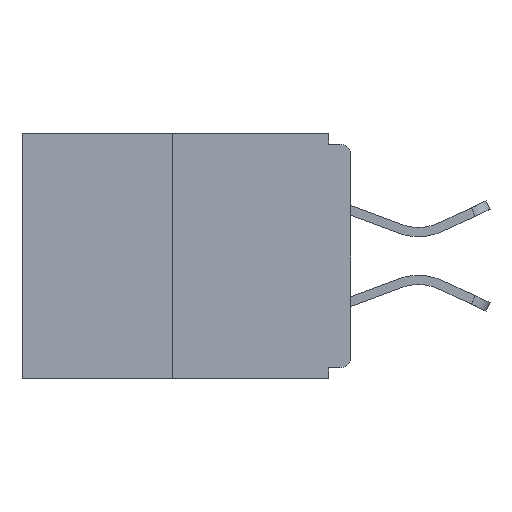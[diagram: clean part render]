
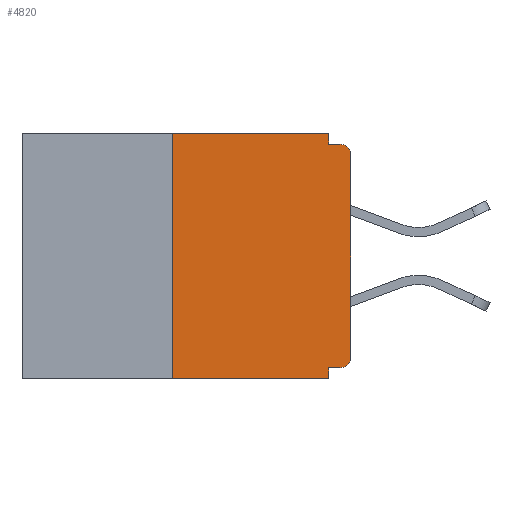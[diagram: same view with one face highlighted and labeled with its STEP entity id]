
A CAD part, left-side view. The second image highlights one B-rep face of the part: STEP entity #4820.
In plain terms, the highlighted planar face has unit normal (-1, 0, 0).
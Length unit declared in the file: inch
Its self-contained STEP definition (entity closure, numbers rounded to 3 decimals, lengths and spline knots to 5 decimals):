
#71 = LINE ( 'NONE', #4226, #3822 ) ;
#185 = VECTOR ( 'NONE', #7769, 39.37008 ) ;
#435 = EDGE_CURVE ( 'NONE', #2925, #9922, #7428, .T. ) ;
#478 = ORIENTED_EDGE ( 'NONE', *, *, #12668, .T. ) ;
#519 = VERTEX_POINT ( 'NONE', #4564 ) ;
#611 = ORIENTED_EDGE ( 'NONE', *, *, #435, .T. ) ;
#626 = CARTESIAN_POINT ( 'NONE',  ( 0., 0.46, -0.343 ) ) ;
#725 = ORIENTED_EDGE ( 'NONE', *, *, #7886, .F. ) ;
#737 = VECTOR ( 'NONE', #5332, 39.37008 ) ;
#765 = DIRECTION ( 'NONE',  ( 0., 0., -1. ) ) ;
#860 = DIRECTION ( 'NONE',  ( 1., 0., 0. ) ) ;
#923 = ORIENTED_EDGE ( 'NONE', *, *, #10808, .F. ) ;
#1026 = CARTESIAN_POINT ( 'NONE',  ( 0., 0., -0.03 ) ) ;
#1779 = EDGE_CURVE ( 'NONE', #11652, #10095, #10663, .T. ) ;
#2315 = DIRECTION ( 'NONE',  ( 0., -1., 0. ) ) ;
#2351 = EDGE_CURVE ( 'NONE', #9922, #11652, #6791, .T. ) ;
#2826 = EDGE_LOOP ( 'NONE', ( #10183, #725, #478, #5911, #923, #611, #11183, #9332, #3282, #5860 ) ) ;
#2859 = CARTESIAN_POINT ( 'NONE',  ( 0., 0.031, 0. ) ) ;
#2925 = VERTEX_POINT ( 'NONE', #9505 ) ;
#2957 = FACE_OUTER_BOUND ( 'NONE', #2826, .T. ) ;
#3062 = AXIS2_PLACEMENT_3D ( 'NONE', #10218, #860, #7151 ) ;
#3282 = ORIENTED_EDGE ( 'NONE', *, *, #10199, .F. ) ;
#3587 = CARTESIAN_POINT ( 'NONE',  ( 0., 0., -0.313 ) ) ;
#3663 = DIRECTION ( 'NONE',  ( 0., -1., 0. ) ) ;
#3822 = VECTOR ( 'NONE', #7380, 39.37008 ) ;
#3829 = CARTESIAN_POINT ( 'NONE',  ( 0., 0.031, -0.343 ) ) ;
#3863 = VERTEX_POINT ( 'NONE', #10115 ) ;
#3864 = EDGE_CURVE ( 'NONE', #519, #10175, #6966, .T. ) ;
#4024 = DIRECTION ( 'NONE',  ( 0., 0., -1. ) ) ;
#4149 = CARTESIAN_POINT ( 'NONE',  ( 0., 0.031, -0.328 ) ) ;
#4226 = CARTESIAN_POINT ( 'NONE',  ( 0., 0., -0.015 ) ) ;
#4564 = CARTESIAN_POINT ( 'NONE',  ( 0., 0.031, 0. ) ) ;
#4583 = CARTESIAN_POINT ( 'NONE',  ( 0., 0.46, 0. ) ) ;
#4603 = CARTESIAN_POINT ( 'NONE',  ( 0., 0., -0.328 ) ) ;
#4730 = VECTOR ( 'NONE', #3663, 39.37008 ) ;
#4741 = LINE ( 'NONE', #4603, #7760 ) ;
#4764 = AXIS2_PLACEMENT_3D ( 'NONE', #7542, #11689, #12145 ) ;
#4820 = ADVANCED_FACE ( 'NONE', ( #2957 ), #12244, .F. ) ;
#5332 = DIRECTION ( 'NONE',  ( 0., 0., 1. ) ) ;
#5860 = ORIENTED_EDGE ( 'NONE', *, *, #3864, .F. ) ;
#5911 = ORIENTED_EDGE ( 'NONE', *, *, #7331, .F. ) ;
#6486 = VERTEX_POINT ( 'NONE', #4149 ) ;
#6642 = CARTESIAN_POINT ( 'NONE',  ( 0., 0.25, 0. ) ) ;
#6791 = LINE ( 'NONE', #9806, #185 ) ;
#6966 = LINE ( 'NONE', #2859, #11855 ) ;
#6979 = DIRECTION ( 'NONE',  ( 0., 0., -1. ) ) ;
#7151 = DIRECTION ( 'NONE',  ( 0., 0., -1. ) ) ;
#7331 = EDGE_CURVE ( 'NONE', #6486, #12610, #12087, .T. ) ;
#7380 = DIRECTION ( 'NONE',  ( 0., -1., 0. ) ) ;
#7428 = CIRCLE ( 'NONE', #8514, 0.015 ) ;
#7466 = LINE ( 'NONE', #4583, #9460 ) ;
#7514 = CARTESIAN_POINT ( 'NONE',  ( 0., 0.25, 0. ) ) ;
#7542 = CARTESIAN_POINT ( 'NONE',  ( 0., 0.015, -0.03 ) ) ;
#7760 = VECTOR ( 'NONE', #12916, 39.37008 ) ;
#7769 = DIRECTION ( 'NONE',  ( 0., 0., 1. ) ) ;
#7886 = EDGE_CURVE ( 'NONE', #3863, #10737, #8539, .T. ) ;
#8077 = DIRECTION ( 'NONE',  ( -1., 0., 0. ) ) ;
#8514 = AXIS2_PLACEMENT_3D ( 'NONE', #9082, #8077, #4024 ) ;
#8539 = LINE ( 'NONE', #7514, #737 ) ;
#9082 = CARTESIAN_POINT ( 'NONE',  ( 0., 0.015, -0.313 ) ) ;
#9228 = EDGE_CURVE ( 'NONE', #10737, #519, #7466, .T. ) ;
#9332 = ORIENTED_EDGE ( 'NONE', *, *, #1779, .T. ) ;
#9422 = CARTESIAN_POINT ( 'NONE',  ( 0., 0.015, -0.015 ) ) ;
#9460 = VECTOR ( 'NONE', #2315, 39.37008 ) ;
#9505 = CARTESIAN_POINT ( 'NONE',  ( 0., 0.015, -0.328 ) ) ;
#9806 = CARTESIAN_POINT ( 'NONE',  ( 0., 0., 0. ) ) ;
#9922 = VERTEX_POINT ( 'NONE', #3587 ) ;
#10095 = VERTEX_POINT ( 'NONE', #9422 ) ;
#10115 = CARTESIAN_POINT ( 'NONE',  ( 0., 0.25, -0.343 ) ) ;
#10175 = VERTEX_POINT ( 'NONE', #10706 ) ;
#10183 = ORIENTED_EDGE ( 'NONE', *, *, #9228, .F. ) ;
#10199 = EDGE_CURVE ( 'NONE', #10175, #10095, #71, .T. ) ;
#10218 = CARTESIAN_POINT ( 'NONE',  ( 0., 0.46, 0. ) ) ;
#10663 = CIRCLE ( 'NONE', #4764, 0.015 ) ;
#10706 = CARTESIAN_POINT ( 'NONE',  ( 0., 0.031, -0.015 ) ) ;
#10737 = VERTEX_POINT ( 'NONE', #6642 ) ;
#10808 = EDGE_CURVE ( 'NONE', #2925, #6486, #4741, .T. ) ;
#10960 = VECTOR ( 'NONE', #6979, 39.37008 ) ;
#11183 = ORIENTED_EDGE ( 'NONE', *, *, #2351, .T. ) ;
#11652 = VERTEX_POINT ( 'NONE', #1026 ) ;
#11669 = CARTESIAN_POINT ( 'NONE',  ( 0., 0.031, -0.343 ) ) ;
#11689 = DIRECTION ( 'NONE',  ( -1., 0., 0. ) ) ;
#11855 = VECTOR ( 'NONE', #765, 39.37008 ) ;
#12087 = LINE ( 'NONE', #3829, #10960 ) ;
#12145 = DIRECTION ( 'NONE',  ( 0., 0., -1. ) ) ;
#12244 = PLANE ( 'NONE',  #3062 ) ;
#12279 = LINE ( 'NONE', #626, #4730 ) ;
#12610 = VERTEX_POINT ( 'NONE', #11669 ) ;
#12668 = EDGE_CURVE ( 'NONE', #3863, #12610, #12279, .T. ) ;
#12916 = DIRECTION ( 'NONE',  ( 0., 1., 0. ) ) ;
